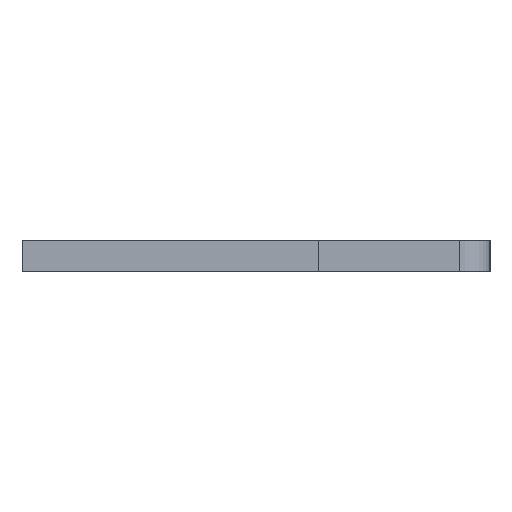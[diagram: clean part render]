
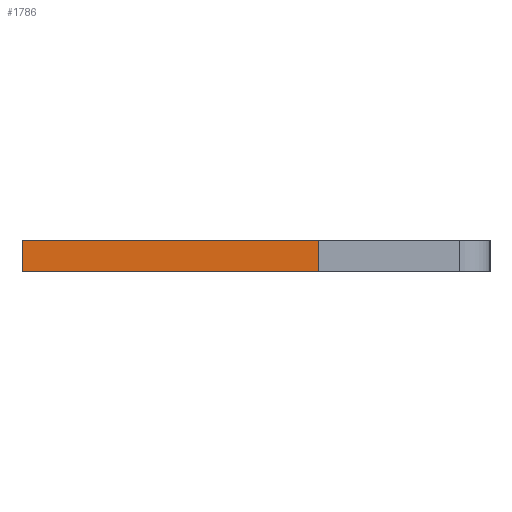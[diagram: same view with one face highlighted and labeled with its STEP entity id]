
A CAD part, left-side view. The second image highlights one B-rep face of the part: STEP entity #1786.
In plain terms, the highlighted face is planar.
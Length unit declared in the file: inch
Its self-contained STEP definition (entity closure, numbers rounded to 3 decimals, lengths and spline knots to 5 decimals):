
#84 = EDGE_CURVE ( 'NONE', #1497, #1575, #1778, .T. ) ;
#261 = ORIENTED_EDGE ( 'NONE', *, *, #1155, .T. ) ;
#288 = LINE ( 'NONE', #323, #1081 ) ;
#323 = CARTESIAN_POINT ( 'NONE',  ( 0.01, 0.15, -0.04 ) ) ;
#332 = CARTESIAN_POINT ( 'NONE',  ( -0.01, 0.15, -0.04 ) ) ;
#402 = LINE ( 'NONE', #898, #817 ) ;
#416 = ORIENTED_EDGE ( 'NONE', *, *, #902, .T. ) ;
#440 = VERTEX_POINT ( 'NONE', #1711 ) ;
#473 = DIRECTION ( 'NONE',  ( 0., 0., 1. ) ) ;
#746 = CARTESIAN_POINT ( 'NONE',  ( 0.01, 0.15, -0.04 ) ) ;
#778 = VERTEX_POINT ( 'NONE', #1421 ) ;
#791 = CARTESIAN_POINT ( 'NONE',  ( 0.01, 0.15, -0.04 ) ) ;
#817 = VECTOR ( 'NONE', #1779, 39.37008 ) ;
#819 = CARTESIAN_POINT ( 'NONE',  ( -0.01, 0.15, -0.04 ) ) ;
#891 = EDGE_CURVE ( 'NONE', #778, #1497, #288, .T. ) ;
#898 = CARTESIAN_POINT ( 'NONE',  ( 0.01, -0.04, -0.04 ) ) ;
#902 = EDGE_CURVE ( 'NONE', #440, #1575, #997, .T. ) ;
#997 = LINE ( 'NONE', #332, #1217 ) ;
#1081 = VECTOR ( 'NONE', #1742, 39.37008 ) ;
#1082 = CARTESIAN_POINT ( 'NONE',  ( 0.01, 0.15, -0.04 ) ) ;
#1139 = DIRECTION ( 'NONE',  ( 1., 0., 0. ) ) ;
#1155 = EDGE_CURVE ( 'NONE', #778, #440, #402, .T. ) ;
#1171 = DIRECTION ( 'NONE',  ( 0., 1., 0. ) ) ;
#1217 = VECTOR ( 'NONE', #1171, 39.37008 ) ;
#1233 = EDGE_LOOP ( 'NONE', ( #416, #1428, #1553, #261 ) ) ;
#1248 = AXIS2_PLACEMENT_3D ( 'NONE', #746, #473, #1139 ) ;
#1376 = VECTOR ( 'NONE', #1507, 39.37008 ) ;
#1421 = CARTESIAN_POINT ( 'NONE',  ( 0.01, -0.04, -0.04 ) ) ;
#1428 = ORIENTED_EDGE ( 'NONE', *, *, #84, .F. ) ;
#1479 = FACE_OUTER_BOUND ( 'NONE', #1233, .T. ) ;
#1497 = VERTEX_POINT ( 'NONE', #791 ) ;
#1507 = DIRECTION ( 'NONE',  ( -1., 0., 0. ) ) ;
#1553 = ORIENTED_EDGE ( 'NONE', *, *, #891, .F. ) ;
#1575 = VERTEX_POINT ( 'NONE', #819 ) ;
#1622 = PLANE ( 'NONE',  #1248 ) ;
#1711 = CARTESIAN_POINT ( 'NONE',  ( -0.01, -0.04, -0.04 ) ) ;
#1742 = DIRECTION ( 'NONE',  ( 0., 1., 0. ) ) ;
#1778 = LINE ( 'NONE', #1082, #1376 ) ;
#1779 = DIRECTION ( 'NONE',  ( -1., 0., 0. ) ) ;
#1786 = ADVANCED_FACE ( 'NONE', ( #1479 ), #1622, .F. ) ;
